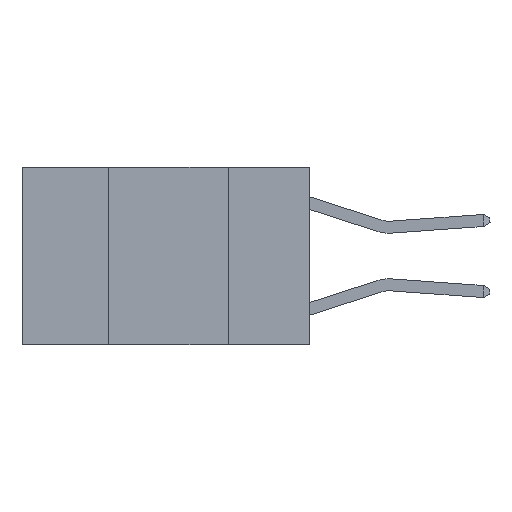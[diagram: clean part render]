
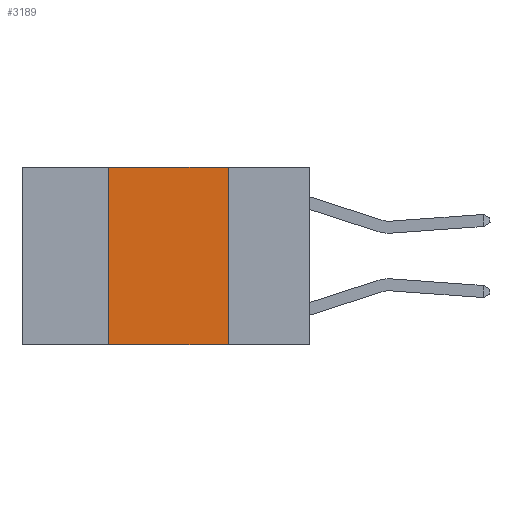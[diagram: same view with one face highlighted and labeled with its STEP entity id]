
A CAD part, left-side view. The second image highlights one B-rep face of the part: STEP entity #3189.
In plain terms, the highlighted planar face has unit normal (-1, 0, 0).
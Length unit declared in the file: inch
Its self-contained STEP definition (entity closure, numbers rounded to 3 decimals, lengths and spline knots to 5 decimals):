
#81 = AXIS2_PLACEMENT_3D ( 'NONE', #6423, #6054, #6037 ) ;
#275 = LINE ( 'NONE', #9683, #8770 ) ;
#835 = DIRECTION ( 'NONE',  ( 0., -1., 0. ) ) ;
#966 = CARTESIAN_POINT ( 'NONE',  ( 0., 0.42, -0.37 ) ) ;
#1707 = FACE_OUTER_BOUND ( 'NONE', #4066, .T. ) ;
#1973 = ORIENTED_EDGE ( 'NONE', *, *, #4469, .T. ) ;
#2187 = DIRECTION ( 'NONE',  ( 0., 0., -1. ) ) ;
#2456 = DIRECTION ( 'NONE',  ( 0., 0., 1. ) ) ;
#2496 = CARTESIAN_POINT ( 'NONE',  ( 0., 0.42, 0. ) ) ;
#3189 = ADVANCED_FACE ( 'NONE', ( #1707 ), #6058, .F. ) ;
#3213 = VECTOR ( 'NONE', #6774, 39.37008 ) ;
#3478 = VERTEX_POINT ( 'NONE', #966 ) ;
#3887 = ORIENTED_EDGE ( 'NONE', *, *, #4622, .F. ) ;
#4066 = EDGE_LOOP ( 'NONE', ( #7924, #3887, #8168, #1973 ) ) ;
#4197 = VERTEX_POINT ( 'NONE', #7733 ) ;
#4334 = EDGE_CURVE ( 'NONE', #8415, #4197, #6291, .T. ) ;
#4469 = EDGE_CURVE ( 'NONE', #3478, #4197, #275, .T. ) ;
#4622 = EDGE_CURVE ( 'NONE', #8334, #8415, #5420, .T. ) ;
#4821 = VECTOR ( 'NONE', #2456, 39.37008 ) ;
#5420 = LINE ( 'NONE', #9862, #3213 ) ;
#6037 = DIRECTION ( 'NONE',  ( 0., 0., -1. ) ) ;
#6054 = DIRECTION ( 'NONE',  ( 1., 0., 0. ) ) ;
#6058 = PLANE ( 'NONE',  #81 ) ;
#6291 = LINE ( 'NONE', #8630, #8161 ) ;
#6423 = CARTESIAN_POINT ( 'NONE',  ( 0., 0.6, 0. ) ) ;
#6716 = LINE ( 'NONE', #9646, #4821 ) ;
#6774 = DIRECTION ( 'NONE',  ( 0., -1., 0. ) ) ;
#7733 = CARTESIAN_POINT ( 'NONE',  ( 0., 0.17, -0.37 ) ) ;
#7924 = ORIENTED_EDGE ( 'NONE', *, *, #4334, .F. ) ;
#8161 = VECTOR ( 'NONE', #2187, 39.37008 ) ;
#8168 = ORIENTED_EDGE ( 'NONE', *, *, #10145, .F. ) ;
#8334 = VERTEX_POINT ( 'NONE', #2496 ) ;
#8415 = VERTEX_POINT ( 'NONE', #9752 ) ;
#8630 = CARTESIAN_POINT ( 'NONE',  ( 0., 0.17, 0. ) ) ;
#8770 = VECTOR ( 'NONE', #835, 39.37008 ) ;
#9646 = CARTESIAN_POINT ( 'NONE',  ( 0., 0.42, 0. ) ) ;
#9683 = CARTESIAN_POINT ( 'NONE',  ( 0., 0.6, -0.37 ) ) ;
#9752 = CARTESIAN_POINT ( 'NONE',  ( 0., 0.17, 0. ) ) ;
#9862 = CARTESIAN_POINT ( 'NONE',  ( 0., 0.6, 0. ) ) ;
#10145 = EDGE_CURVE ( 'NONE', #3478, #8334, #6716, .T. ) ;
